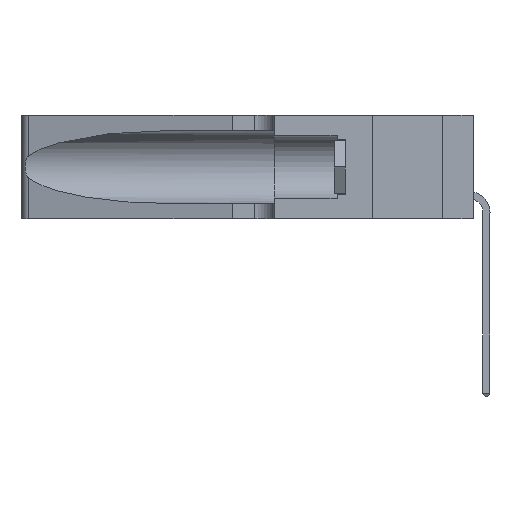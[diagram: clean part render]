
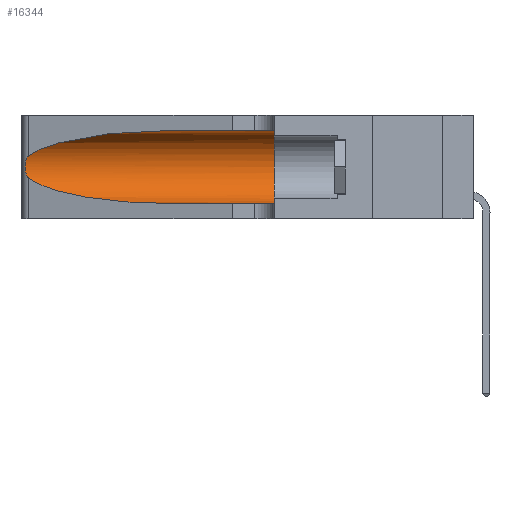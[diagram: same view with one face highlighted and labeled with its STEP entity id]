
A CAD part, left-side view. The second image highlights one B-rep face of the part: STEP entity #16344.
In plain terms, the highlighted cylindrical face has radius 3.308 mm (diameter 6.617 mm), a partial arc.
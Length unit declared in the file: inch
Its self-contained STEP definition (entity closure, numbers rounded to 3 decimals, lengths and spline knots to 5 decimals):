
#1148 = CARTESIAN_POINT ( 'NONE',  ( 0.2373, 1.15595, 0.28018 ) ) ;
#2724 = DIRECTION ( 'NONE',  ( 0., 1., 0. ) ) ;
#2892 = CARTESIAN_POINT ( 'NONE',  ( 0.25854, 1.2359, 0.20912 ) ) ;
#3574 = CARTESIAN_POINT ( 'NONE',  ( 0.25789, 1.23486, 0.15765 ) ) ;
#3591 = B_SPLINE_CURVE_WITH_KNOTS ( 'NONE', 3,
 ( #30356, #29885, #5472, #24490, #2892, #8302, #30107, #20042, #3795, #6416, #3574, #33405, #22794, #6530 ),
 .UNSPECIFIED., .F., .F.,
 ( 4, 2, 2, 2, 2, 2, 4 ),
 ( 0., 0.00027, 0.00053, 0.00107, 0.0016, 0.00187, 0.00214 ),
 .UNSPECIFIED. ) ;
#3795 = CARTESIAN_POINT ( 'NONE',  ( 0.26017, 1.23833, 0.17102 ) ) ;
#3978 = CARTESIAN_POINT ( 'NONE',  ( 0.18966, 0.96281, 0.31525 ) ) ;
#4458 = CARTESIAN_POINT ( 'NONE',  ( 0.1305, 0.35, 0.31525 ) ) ;
#4703 = EDGE_CURVE ( 'NONE', #31100, #21760, #19261, .T. ) ;
#5472 = CARTESIAN_POINT ( 'NONE',  ( 0.25639, 1.23184, 0.21858 ) ) ;
#5922 = CARTESIAN_POINT ( 'NONE',  ( 0.1305, 1.61858, 0.185 ) ) ;
#6416 = CARTESIAN_POINT ( 'NONE',  ( 0.25856, 1.23593, 0.16098 ) ) ;
#6530 = CARTESIAN_POINT ( 'NONE',  ( 0.25487, 1.22718, 0.14631 ) ) ;
#6720 = CARTESIAN_POINT ( 'NONE',  ( 0.25487, 1.22718, 0.22369 ) ) ;
#6770 = ORIENTED_EDGE ( 'NONE', *, *, #25351, .F. ) ;
#7892 = CARTESIAN_POINT ( 'NONE',  ( 0.25487, 1.22718, 0.22369 ) ) ;
#8302 = CARTESIAN_POINT ( 'NONE',  ( 0.26018, 1.23835, 0.19895 ) ) ;
#8911 = ORIENTED_EDGE ( 'NONE', *, *, #4703, .T. ) ;
#10664 = FACE_OUTER_BOUND ( 'NONE', #27928, .T. ) ;
#10751 = DIRECTION ( 'NONE',  ( 0., 0., 1. ) ) ;
#11956 = DIRECTION ( 'NONE',  ( 0., -1., 0. ) ) ;
#12036 = VERTEX_POINT ( 'NONE', #31981 ) ;
#13875 = ORIENTED_EDGE ( 'NONE', *, *, #14055, .F. ) ;
#14055 = EDGE_CURVE ( 'NONE', #12036, #17710, #17354, .T. ) ;
#14449 = DIRECTION ( 'NONE',  ( 0., -1., 0. ) ) ;
#15524 = CARTESIAN_POINT ( 'NONE',  ( 0.2373, 1.15595, 0.08982 ) ) ;
#16292 = ORIENTED_EDGE ( 'NONE', *, *, #23066, .T. ) ;
#16344 = ADVANCED_FACE ( 'NONE', ( #10664 ), #22578, .F. ) ;
#16499 = VECTOR ( 'NONE', #11956, 39.37008 ) ;
#17124 = ORIENTED_EDGE ( 'NONE', *, *, #33766, .T. ) ;
#17190 = DIRECTION ( 'NONE',  ( 0., 0., -1. ) ) ;
#17354 = LINE ( 'NONE', #22784, #16499 ) ;
#17710 = VERTEX_POINT ( 'NONE', #4458 ) ;
#17730 =( BOUNDED_CURVE ( )  B_SPLINE_CURVE ( 3, ( #24205, #15524, #21098, #18266 ),
 .UNSPECIFIED., .F., .F. ) 
 B_SPLINE_CURVE_WITH_KNOTS ( ( 4, 4 ),
 ( 3.44316, 4.71239 ),
 .UNSPECIFIED. ) 
 CURVE ( )  GEOMETRIC_REPRESENTATION_ITEM ( )  RATIONAL_B_SPLINE_CURVE ( ( 1., 0.87, 0.87, 1. ) ) 
 REPRESENTATION_ITEM ( '' )  );
#18266 = CARTESIAN_POINT ( 'NONE',  ( 0.1305, 0.72297, 0.05475 ) ) ;
#19213 = CARTESIAN_POINT ( 'NONE',  ( 0.1305, 0.35, 0.05475 ) ) ;
#19261 = LINE ( 'NONE', #22123, #32075 ) ;
#20042 = CARTESIAN_POINT ( 'NONE',  ( 0.26075, 1.23896, 0.178 ) ) ;
#20801 =( BOUNDED_CURVE ( )  B_SPLINE_CURVE ( 3, ( #22990, #3978, #1148, #6720 ),
 .UNSPECIFIED., .F., .T. ) 
 B_SPLINE_CURVE_WITH_KNOTS ( ( 4, 4 ),
 ( 1.5708, 2.84003 ),
 .UNSPECIFIED. ) 
 CURVE ( )  GEOMETRIC_REPRESENTATION_ITEM ( )  RATIONAL_B_SPLINE_CURVE ( ( 1., 0.87, 0.87, 1. ) ) 
 REPRESENTATION_ITEM ( '' )  );
#21098 = CARTESIAN_POINT ( 'NONE',  ( 0.18966, 0.96281, 0.05475 ) ) ;
#21760 = VERTEX_POINT ( 'NONE', #19213 ) ;
#21885 = DIRECTION ( 'NONE',  ( 0., -1., 0. ) ) ;
#22123 = CARTESIAN_POINT ( 'NONE',  ( 0.1305, 1.61858, 0.05475 ) ) ;
#22578 = CYLINDRICAL_SURFACE ( 'NONE', #33690, 0.13025 ) ;
#22650 = VERTEX_POINT ( 'NONE', #22719 ) ;
#22719 = CARTESIAN_POINT ( 'NONE',  ( 0.25487, 1.22718, 0.14631 ) ) ;
#22784 = CARTESIAN_POINT ( 'NONE',  ( 0.1305, 1.61858, 0.31525 ) ) ;
#22794 = CARTESIAN_POINT ( 'NONE',  ( 0.25555, 1.22993, 0.14849 ) ) ;
#22990 = CARTESIAN_POINT ( 'NONE',  ( 0.1305, 0.72297, 0.31525 ) ) ;
#23066 = EDGE_CURVE ( 'NONE', #31076, #22650, #3591, .T. ) ;
#24205 = CARTESIAN_POINT ( 'NONE',  ( 0.25487, 1.22718, 0.14631 ) ) ;
#24316 = CARTESIAN_POINT ( 'NONE',  ( 0.1305, 0.35, 0.185 ) ) ;
#24490 = CARTESIAN_POINT ( 'NONE',  ( 0.25787, 1.23484, 0.2124 ) ) ;
#25351 = EDGE_CURVE ( 'NONE', #17710, #21760, #29621, .T. ) ;
#26572 = CARTESIAN_POINT ( 'NONE',  ( 0.1305, 0.72297, 0.05475 ) ) ;
#26801 = ORIENTED_EDGE ( 'NONE', *, *, #33403, .T. ) ;
#27928 = EDGE_LOOP ( 'NONE', ( #17124, #16292, #26801, #8911, #6770, #13875 ) ) ;
#28904 = AXIS2_PLACEMENT_3D ( 'NONE', #24316, #2724, #10751 ) ;
#29621 = CIRCLE ( 'NONE', #28904, 0.13025 ) ;
#29885 = CARTESIAN_POINT ( 'NONE',  ( 0.25555, 1.22994, 0.2215 ) ) ;
#30107 = CARTESIAN_POINT ( 'NONE',  ( 0.26075, 1.23896, 0.19203 ) ) ;
#30356 = CARTESIAN_POINT ( 'NONE',  ( 0.25487, 1.22718, 0.22369 ) ) ;
#31076 = VERTEX_POINT ( 'NONE', #7892 ) ;
#31100 = VERTEX_POINT ( 'NONE', #26572 ) ;
#31981 = CARTESIAN_POINT ( 'NONE',  ( 0.1305, 0.72297, 0.31525 ) ) ;
#32075 = VECTOR ( 'NONE', #21885, 39.37008 ) ;
#33403 = EDGE_CURVE ( 'NONE', #22650, #31100, #17730, .T. ) ;
#33405 = CARTESIAN_POINT ( 'NONE',  ( 0.25639, 1.23186, 0.15144 ) ) ;
#33690 = AXIS2_PLACEMENT_3D ( 'NONE', #5922, #14449, #17190 ) ;
#33766 = EDGE_CURVE ( 'NONE', #12036, #31076, #20801, .T. ) ;
